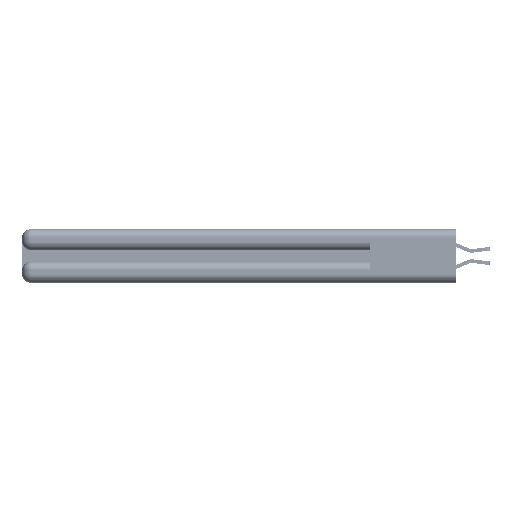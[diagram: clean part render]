
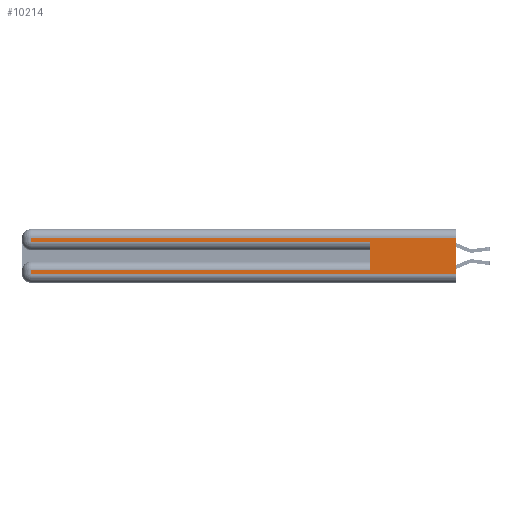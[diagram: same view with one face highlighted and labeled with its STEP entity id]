
A CAD part, left-side view. The second image highlights one B-rep face of the part: STEP entity #10214.
In plain terms, the highlighted planar face has unit normal (-1, 0, 0).
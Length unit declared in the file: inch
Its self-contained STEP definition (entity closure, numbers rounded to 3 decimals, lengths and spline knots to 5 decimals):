
#91 = VERTEX_POINT ( 'NONE', #5919 ) ;
#102 = VECTOR ( 'NONE', #48584, 39.37008 ) ;
#952 = LINE ( 'NONE', #39695, #21653 ) ;
#957 = VECTOR ( 'NONE', #1249, 39.37008 ) ;
#1249 = DIRECTION ( 'NONE',  ( 0., 0., -1. ) ) ;
#1754 = CARTESIAN_POINT ( 'NONE',  ( 0., 0., 0.06 ) ) ;
#2746 = LINE ( 'NONE', #34787, #8024 ) ;
#2878 = VERTEX_POINT ( 'NONE', #45532 ) ;
#3995 = ORIENTED_EDGE ( 'NONE', *, *, #28004, .F. ) ;
#4499 = VERTEX_POINT ( 'NONE', #28753 ) ;
#5919 = CARTESIAN_POINT ( 'NONE',  ( 0., 2.94, 0.285 ) ) ;
#6969 = DIRECTION ( 'NONE',  ( 1., 0., 0. ) ) ;
#7415 = EDGE_CURVE ( 'NONE', #21805, #15329, #24030, .T. ) ;
#8024 = VECTOR ( 'NONE', #26124, 39.37008 ) ;
#8088 = VERTEX_POINT ( 'NONE', #51184 ) ;
#10214 = ADVANCED_FACE ( 'NONE', ( #43237 ), #52822, .F. ) ;
#10899 = VECTOR ( 'NONE', #19624, 39.37008 ) ;
#13085 = VECTOR ( 'NONE', #18221, 39.37008 ) ;
#14114 = ORIENTED_EDGE ( 'NONE', *, *, #33571, .T. ) ;
#15266 = VERTEX_POINT ( 'NONE', #50847 ) ;
#15329 = VERTEX_POINT ( 'NONE', #1754 ) ;
#15522 = CARTESIAN_POINT ( 'NONE',  ( 0., 0., 0.37 ) ) ;
#16198 = EDGE_CURVE ( 'NONE', #2878, #4499, #39538, .T. ) ;
#16738 = LINE ( 'NONE', #44494, #10899 ) ;
#17149 = AXIS2_PLACEMENT_3D ( 'NONE', #15522, #6969, #19293 ) ;
#18221 = DIRECTION ( 'NONE',  ( 0., -1., 0. ) ) ;
#18883 = EDGE_LOOP ( 'NONE', ( #32886, #22041, #43439, #38883, #3995, #31117, #14114, #51222 ) ) ;
#19293 = DIRECTION ( 'NONE',  ( 0., 0., -1. ) ) ;
#19582 = CARTESIAN_POINT ( 'NONE',  ( 0., 0., 0.31 ) ) ;
#19624 = DIRECTION ( 'NONE',  ( 0., 0., -1. ) ) ;
#19778 = DIRECTION ( 'NONE',  ( 0., 0., -1. ) ) ;
#21367 = LINE ( 'NONE', #34978, #29761 ) ;
#21653 = VECTOR ( 'NONE', #44019, 39.37008 ) ;
#21805 = VERTEX_POINT ( 'NONE', #49983 ) ;
#21854 = CARTESIAN_POINT ( 'NONE',  ( 0., 0., 0.37 ) ) ;
#21981 = EDGE_CURVE ( 'NONE', #2878, #15329, #23608, .T. ) ;
#22041 = ORIENTED_EDGE ( 'NONE', *, *, #16198, .T. ) ;
#23608 = LINE ( 'NONE', #21854, #957 ) ;
#23832 = EDGE_CURVE ( 'NONE', #91, #15266, #21367, .T. ) ;
#24030 = LINE ( 'NONE', #42940, #13085 ) ;
#26124 = DIRECTION ( 'NONE',  ( 0., 1., 0. ) ) ;
#28004 = EDGE_CURVE ( 'NONE', #48266, #15266, #952, .T. ) ;
#28231 = VECTOR ( 'NONE', #19778, 39.37008 ) ;
#28753 = CARTESIAN_POINT ( 'NONE',  ( 0., 2.94, 0.31 ) ) ;
#29761 = VECTOR ( 'NONE', #31002, 39.37008 ) ;
#31002 = DIRECTION ( 'NONE',  ( 0., -1., 0. ) ) ;
#31117 = ORIENTED_EDGE ( 'NONE', *, *, #36297, .T. ) ;
#32886 = ORIENTED_EDGE ( 'NONE', *, *, #21981, .F. ) ;
#33571 = EDGE_CURVE ( 'NONE', #8088, #21805, #45642, .T. ) ;
#34787 = CARTESIAN_POINT ( 'NONE',  ( 0., 0., 0.085 ) ) ;
#34809 = CARTESIAN_POINT ( 'NONE',  ( 0., 0.6, 0.085 ) ) ;
#34978 = CARTESIAN_POINT ( 'NONE',  ( 0., 0., 0.285 ) ) ;
#36297 = EDGE_CURVE ( 'NONE', #48266, #8088, #2746, .T. ) ;
#38883 = ORIENTED_EDGE ( 'NONE', *, *, #23832, .T. ) ;
#38894 = CARTESIAN_POINT ( 'NONE',  ( 0., 2.94, 0.37 ) ) ;
#39538 = LINE ( 'NONE', #19582, #102 ) ;
#39671 = EDGE_CURVE ( 'NONE', #4499, #91, #16738, .T. ) ;
#39695 = CARTESIAN_POINT ( 'NONE',  ( 0., 0.6, 0.145 ) ) ;
#42940 = CARTESIAN_POINT ( 'NONE',  ( 0., 0., 0.06 ) ) ;
#43237 = FACE_OUTER_BOUND ( 'NONE', #18883, .T. ) ;
#43439 = ORIENTED_EDGE ( 'NONE', *, *, #39671, .T. ) ;
#44019 = DIRECTION ( 'NONE',  ( 0., 0., 1. ) ) ;
#44494 = CARTESIAN_POINT ( 'NONE',  ( 0., 2.94, 0.37 ) ) ;
#45532 = CARTESIAN_POINT ( 'NONE',  ( 0., 0., 0.31 ) ) ;
#45642 = LINE ( 'NONE', #38894, #28231 ) ;
#48266 = VERTEX_POINT ( 'NONE', #34809 ) ;
#48584 = DIRECTION ( 'NONE',  ( 0., 1., 0. ) ) ;
#49983 = CARTESIAN_POINT ( 'NONE',  ( 0., 2.94, 0.06 ) ) ;
#50847 = CARTESIAN_POINT ( 'NONE',  ( 0., 0.6, 0.285 ) ) ;
#51184 = CARTESIAN_POINT ( 'NONE',  ( 0., 2.94, 0.085 ) ) ;
#51222 = ORIENTED_EDGE ( 'NONE', *, *, #7415, .T. ) ;
#52822 = PLANE ( 'NONE',  #17149 ) ;
